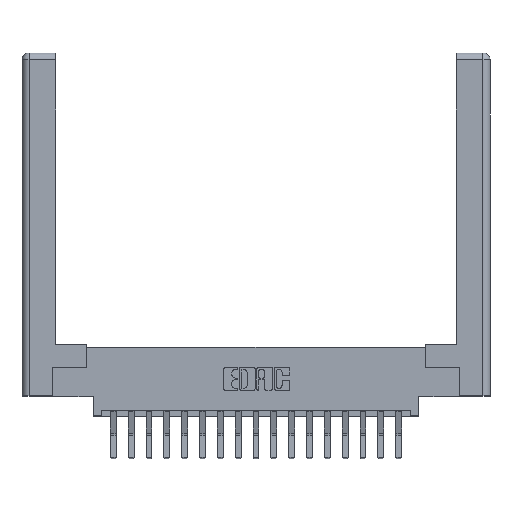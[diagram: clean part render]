
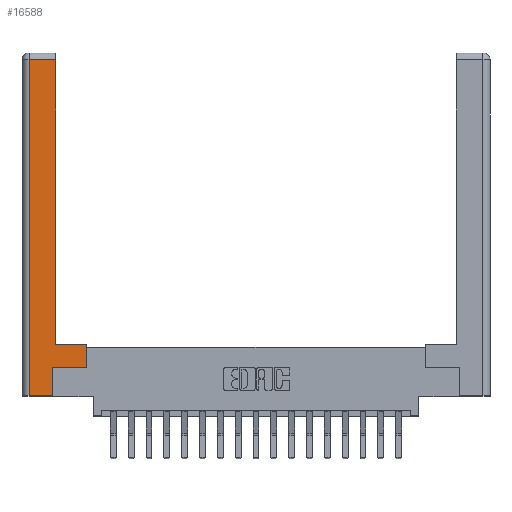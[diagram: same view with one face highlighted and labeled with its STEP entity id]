
A CAD part, top view. The second image highlights one B-rep face of the part: STEP entity #16588.
In plain terms, the highlighted planar face has unit normal (0, 0, 1).
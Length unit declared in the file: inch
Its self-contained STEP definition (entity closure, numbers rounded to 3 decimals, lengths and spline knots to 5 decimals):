
#385 = EDGE_CURVE ( 'NONE', #4512, #12808, #1171, .T. ) ;
#761 = ORIENTED_EDGE ( 'NONE', *, *, #10986, .T. ) ;
#1171 = LINE ( 'NONE', #8715, #1413 ) ;
#1286 = VERTEX_POINT ( 'NONE', #16183 ) ;
#1413 = VECTOR ( 'NONE', #19136, 39.37008 ) ;
#1517 = CARTESIAN_POINT ( 'NONE',  ( 0.565, 0.45, 0. ) ) ;
#2541 = VECTOR ( 'NONE', #4581, 39.37008 ) ;
#2807 = ORIENTED_EDGE ( 'NONE', *, *, #13738, .T. ) ;
#2930 = EDGE_CURVE ( 'NONE', #8105, #1286, #16992, .T. ) ;
#3147 = VECTOR ( 'NONE', #14977, 39.37008 ) ;
#3285 = DIRECTION ( 'NONE',  ( 1., 0., 0. ) ) ;
#3956 = LINE ( 'NONE', #12220, #14206 ) ;
#4172 = CARTESIAN_POINT ( 'NONE',  ( 0.265, 0., 0. ) ) ;
#4303 = DIRECTION ( 'NONE',  ( 0., 1., 0. ) ) ;
#4512 = VERTEX_POINT ( 'NONE', #4172 ) ;
#4573 = CARTESIAN_POINT ( 'NONE',  ( 0.0615, 2.94, 0. ) ) ;
#4581 = DIRECTION ( 'NONE',  ( 0., -1., 0. ) ) ;
#4810 = DIRECTION ( 'NONE',  ( 1., 0., 0. ) ) ;
#6385 = ORIENTED_EDGE ( 'NONE', *, *, #14900, .T. ) ;
#6435 = FACE_OUTER_BOUND ( 'NONE', #13970, .T. ) ;
#6464 = ORIENTED_EDGE ( 'NONE', *, *, #6770, .T. ) ;
#6770 = EDGE_CURVE ( 'NONE', #18972, #8105, #11703, .T. ) ;
#7521 = CARTESIAN_POINT ( 'NONE',  ( 0.295, 0.45, 0. ) ) ;
#7682 = CARTESIAN_POINT ( 'NONE',  ( 0.295, 0.45, 0. ) ) ;
#7705 = DIRECTION ( 'NONE',  ( -1., 0., 0. ) ) ;
#7769 = VECTOR ( 'NONE', #13375, 39.37008 ) ;
#7957 = CARTESIAN_POINT ( 'NONE',  ( 0.0615, 0., 0. ) ) ;
#8105 = VERTEX_POINT ( 'NONE', #7682 ) ;
#8715 = CARTESIAN_POINT ( 'NONE',  ( 0.265, 0.245, 0. ) ) ;
#9076 = VECTOR ( 'NONE', #4303, 39.37008 ) ;
#9317 = PLANE ( 'NONE',  #12113 ) ;
#9333 = CARTESIAN_POINT ( 'NONE',  ( 0.295, 3., 0. ) ) ;
#9425 = ORIENTED_EDGE ( 'NONE', *, *, #385, .T. ) ;
#10169 = LINE ( 'NONE', #4573, #12525 ) ;
#10676 = CARTESIAN_POINT ( 'NONE',  ( 0.0615, 0., 0. ) ) ;
#10775 = ORIENTED_EDGE ( 'NONE', *, *, #14875, .T. ) ;
#10986 = EDGE_CURVE ( 'NONE', #18026, #16647, #14881, .T. ) ;
#11115 = ORIENTED_EDGE ( 'NONE', *, *, #12024, .T. ) ;
#11478 = LINE ( 'NONE', #11951, #13279 ) ;
#11703 = LINE ( 'NONE', #7521, #7769 ) ;
#11907 = DIRECTION ( 'NONE',  ( -1., 0., 0. ) ) ;
#11951 = CARTESIAN_POINT ( 'NONE',  ( 0.565, 0.245, 0. ) ) ;
#12024 = EDGE_CURVE ( 'NONE', #1286, #18026, #10169, .T. ) ;
#12113 = AXIS2_PLACEMENT_3D ( 'NONE', #16519, #18114, #7705 ) ;
#12220 = CARTESIAN_POINT ( 'NONE',  ( 0.265, 0., 0. ) ) ;
#12525 = VECTOR ( 'NONE', #11907, 39.37008 ) ;
#12808 = VERTEX_POINT ( 'NONE', #14043 ) ;
#13279 = VECTOR ( 'NONE', #3285, 39.37008 ) ;
#13375 = DIRECTION ( 'NONE',  ( -1., 0., 0. ) ) ;
#13738 = EDGE_CURVE ( 'NONE', #15397, #18972, #14320, .T. ) ;
#13970 = EDGE_LOOP ( 'NONE', ( #17082, #11115, #761, #6385, #9425, #10775, #2807, #6464 ) ) ;
#14043 = CARTESIAN_POINT ( 'NONE',  ( 0.265, 0.245, 0. ) ) ;
#14206 = VECTOR ( 'NONE', #4810, 39.37008 ) ;
#14320 = LINE ( 'NONE', #1517, #3147 ) ;
#14875 = EDGE_CURVE ( 'NONE', #12808, #15397, #11478, .T. ) ;
#14881 = LINE ( 'NONE', #10676, #2541 ) ;
#14900 = EDGE_CURVE ( 'NONE', #16647, #4512, #3956, .T. ) ;
#14972 = CARTESIAN_POINT ( 'NONE',  ( 0.565, 0.245, 0. ) ) ;
#14977 = DIRECTION ( 'NONE',  ( 0., 1., 0. ) ) ;
#15397 = VERTEX_POINT ( 'NONE', #14972 ) ;
#16183 = CARTESIAN_POINT ( 'NONE',  ( 0.295, 2.94, 0. ) ) ;
#16519 = CARTESIAN_POINT ( 'NONE',  ( 0., 0., 0. ) ) ;
#16588 = ADVANCED_FACE ( 'NONE', ( #6435 ), #9317, .F. ) ;
#16647 = VERTEX_POINT ( 'NONE', #7957 ) ;
#16992 = LINE ( 'NONE', #9333, #9076 ) ;
#17082 = ORIENTED_EDGE ( 'NONE', *, *, #2930, .T. ) ;
#17894 = CARTESIAN_POINT ( 'NONE',  ( 0.565, 0.45, 0. ) ) ;
#18026 = VERTEX_POINT ( 'NONE', #18138 ) ;
#18114 = DIRECTION ( 'NONE',  ( 0., 0., -1. ) ) ;
#18138 = CARTESIAN_POINT ( 'NONE',  ( 0.0615, 2.94, 0. ) ) ;
#18972 = VERTEX_POINT ( 'NONE', #17894 ) ;
#19136 = DIRECTION ( 'NONE',  ( 0., 1., 0. ) ) ;
